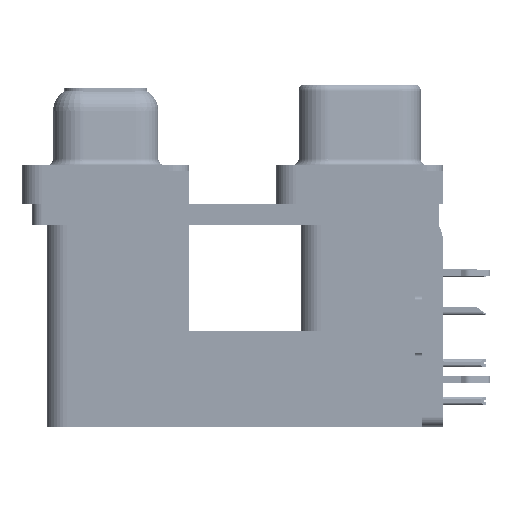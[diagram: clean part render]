
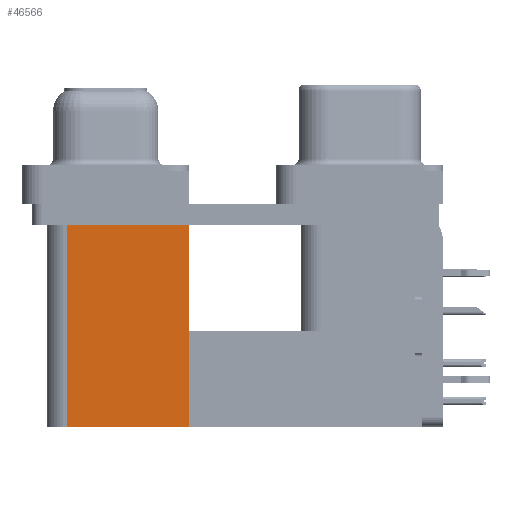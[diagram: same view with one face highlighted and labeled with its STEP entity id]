
A CAD part, left-side view. The second image highlights one B-rep face of the part: STEP entity #46566.
In plain terms, the highlighted planar face has unit normal (-1, 0, 0).
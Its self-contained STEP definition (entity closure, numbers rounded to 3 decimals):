
#6841 = CARTESIAN_POINT ( 'NONE',  ( 3.7, 12.775, -2.5 ) ) ;
#6904 = CARTESIAN_POINT ( 'NONE',  ( 3.7, 12.775, -19.2 ) ) ;
#7308 = EDGE_CURVE ( 'NONE', #50723, #55271, #22131, .T. ) ;
#8841 = DIRECTION ( 'NONE',  ( 0., 1., 0. ) ) ;
#11431 = LINE ( 'NONE', #29772, #16932 ) ;
#11438 = CARTESIAN_POINT ( 'NONE',  ( 3.7, 12.775, -19.2 ) ) ;
#13732 = CARTESIAN_POINT ( 'NONE',  ( 3.7, 21.975, -19.2 ) ) ;
#14424 = LINE ( 'NONE', #11438, #38030 ) ;
#14521 = CARTESIAN_POINT ( 'NONE',  ( 3.7, 12.775, -2.5 ) ) ;
#16453 = ORIENTED_EDGE ( 'NONE', *, *, #7308, .T. ) ;
#16932 = VECTOR ( 'NONE', #47542, 1000. ) ;
#18405 = LINE ( 'NONE', #49324, #42230 ) ;
#19075 = DIRECTION ( 'NONE',  ( 0., 0., 1. ) ) ;
#19082 = VECTOR ( 'NONE', #22974, 1000. ) ;
#22131 = LINE ( 'NONE', #14521, #19082 ) ;
#22974 = DIRECTION ( 'NONE',  ( 0., 1., 0. ) ) ;
#24193 = ORIENTED_EDGE ( 'NONE', *, *, #52216, .F. ) ;
#24940 = DIRECTION ( 'NONE',  ( 1., 0., 0. ) ) ;
#24958 = VERTEX_POINT ( 'NONE', #13732 ) ;
#25393 = CARTESIAN_POINT ( 'NONE',  ( 3.7, 21.975, -2.5 ) ) ;
#29772 = CARTESIAN_POINT ( 'NONE',  ( 3.7, 21.975, -19.2 ) ) ;
#32208 = VERTEX_POINT ( 'NONE', #35146 ) ;
#34626 = ORIENTED_EDGE ( 'NONE', *, *, #35402, .F. ) ;
#35146 = CARTESIAN_POINT ( 'NONE',  ( 3.7, 12.775, -19.2 ) ) ;
#35402 = EDGE_CURVE ( 'NONE', #32208, #24958, #18405, .T. ) ;
#36187 = AXIS2_PLACEMENT_3D ( 'NONE', #6904, #24940, #42130 ) ;
#37193 = FACE_OUTER_BOUND ( 'NONE', #44786, .T. ) ;
#38030 = VECTOR ( 'NONE', #19075, 1000. ) ;
#42130 = DIRECTION ( 'NONE',  ( 0., 0., -1. ) ) ;
#42230 = VECTOR ( 'NONE', #8841, 1000. ) ;
#43044 = EDGE_CURVE ( 'NONE', #32208, #50723, #14424, .T. ) ;
#44786 = EDGE_LOOP ( 'NONE', ( #16453, #24193, #34626, #46245 ) ) ;
#46245 = ORIENTED_EDGE ( 'NONE', *, *, #43044, .T. ) ;
#46566 = ADVANCED_FACE ( 'NONE', ( #37193 ), #54963, .F. ) ;
#47542 = DIRECTION ( 'NONE',  ( 0., 0., 1. ) ) ;
#49324 = CARTESIAN_POINT ( 'NONE',  ( 3.7, 12.775, -19.2 ) ) ;
#50723 = VERTEX_POINT ( 'NONE', #6841 ) ;
#52216 = EDGE_CURVE ( 'NONE', #24958, #55271, #11431, .T. ) ;
#54963 = PLANE ( 'NONE',  #36187 ) ;
#55271 = VERTEX_POINT ( 'NONE', #25393 ) ;
